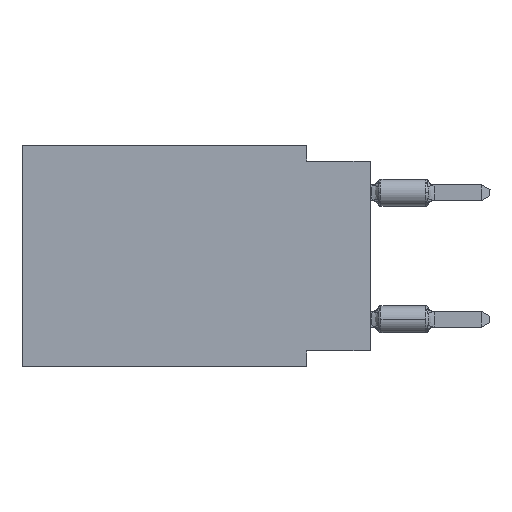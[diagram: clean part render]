
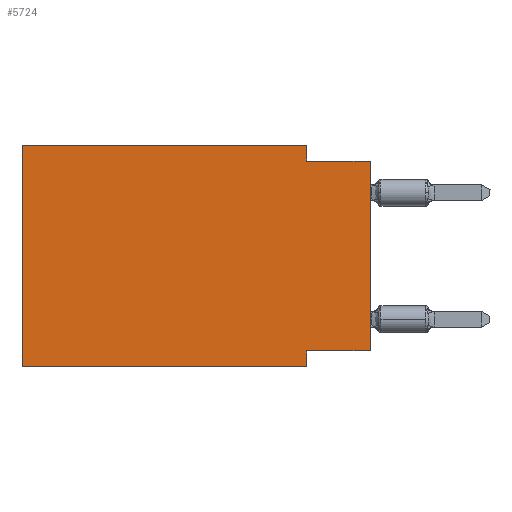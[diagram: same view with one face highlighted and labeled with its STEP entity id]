
A CAD part, left-side view. The second image highlights one B-rep face of the part: STEP entity #5724.
In plain terms, the highlighted planar face has unit normal (-1, 0, 0).
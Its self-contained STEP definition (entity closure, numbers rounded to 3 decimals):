
#1336 = VERTEX_POINT ( 'NONE', #9632 ) ;
#2254 = LINE ( 'NONE', #15727, #28771 ) ;
#2940 = FACE_OUTER_BOUND ( 'NONE', #17958, .T. ) ;
#3119 = ORIENTED_EDGE ( 'NONE', *, *, #3283, .T. ) ;
#3283 = EDGE_CURVE ( 'NONE', #20167, #16165, #27221, .T. ) ;
#3312 = ORIENTED_EDGE ( 'NONE', *, *, #26765, .F. ) ;
#3314 = EDGE_CURVE ( 'NONE', #15516, #1336, #30475, .T. ) ;
#3693 = EDGE_CURVE ( 'NONE', #4203, #21512, #18870, .T. ) ;
#3713 = CARTESIAN_POINT ( 'NONE',  ( 0., 0., -8.255 ) ) ;
#4203 = VERTEX_POINT ( 'NONE', #17099 ) ;
#5093 = DIRECTION ( 'NONE',  ( 0., -1., 0. ) ) ;
#5327 = VECTOR ( 'NONE', #5093, 1000. ) ;
#5641 = EDGE_CURVE ( 'NONE', #21512, #9783, #30757, .T. ) ;
#5724 = ADVANCED_FACE ( 'NONE', ( #2940 ), #10731, .F. ) ;
#7027 = CARTESIAN_POINT ( 'NONE',  ( 0., 2.54, 0. ) ) ;
#7473 = DIRECTION ( 'NONE',  ( 0., -1., 0. ) ) ;
#7504 = VECTOR ( 'NONE', #22390, 1000. ) ;
#7661 = ORIENTED_EDGE ( 'NONE', *, *, #32866, .F. ) ;
#8297 = DIRECTION ( 'NONE',  ( 0., 0., -1. ) ) ;
#9632 = CARTESIAN_POINT ( 'NONE',  ( 0., 2.54, -8.255 ) ) ;
#9783 = VERTEX_POINT ( 'NONE', #26703 ) ;
#10731 = PLANE ( 'NONE',  #22887 ) ;
#11315 = VECTOR ( 'NONE', #22113, 1000. ) ;
#11355 = CARTESIAN_POINT ( 'NONE',  ( 0., 13.97, -8.89 ) ) ;
#11459 = ORIENTED_EDGE ( 'NONE', *, *, #3314, .F. ) ;
#12069 = DIRECTION ( 'NONE',  ( 0., 0., 1. ) ) ;
#12221 = CARTESIAN_POINT ( 'NONE',  ( 0., 0., 0. ) ) ;
#13426 = DIRECTION ( 'NONE',  ( 0., 0., -1. ) ) ;
#13707 = CARTESIAN_POINT ( 'NONE',  ( 0., 13.97, 0. ) ) ;
#14264 = CARTESIAN_POINT ( 'NONE',  ( 0., 0., -8.255 ) ) ;
#14338 = CARTESIAN_POINT ( 'NONE',  ( 0., 13.97, 0. ) ) ;
#15516 = VERTEX_POINT ( 'NONE', #3713 ) ;
#15727 = CARTESIAN_POINT ( 'NONE',  ( 0., 0., -0.635 ) ) ;
#16165 = VERTEX_POINT ( 'NONE', #19003 ) ;
#16587 = LINE ( 'NONE', #14338, #11315 ) ;
#17099 = CARTESIAN_POINT ( 'NONE',  ( 0., 13.97, 0. ) ) ;
#17904 = ORIENTED_EDGE ( 'NONE', *, *, #3693, .F. ) ;
#17958 = EDGE_LOOP ( 'NONE', ( #26863, #3312, #33138, #17904, #29126, #3119, #7661, #11459 ) ) ;
#18870 = LINE ( 'NONE', #13707, #5327 ) ;
#19003 = CARTESIAN_POINT ( 'NONE',  ( 0., 2.54, -8.89 ) ) ;
#19270 = DIRECTION ( 'NONE',  ( 0., 1., 0. ) ) ;
#20006 = EDGE_CURVE ( 'NONE', #15516, #26347, #31041, .T. ) ;
#20167 = VERTEX_POINT ( 'NONE', #26731 ) ;
#20931 = CARTESIAN_POINT ( 'NONE',  ( 0., 0., -0.635 ) ) ;
#21512 = VERTEX_POINT ( 'NONE', #7027 ) ;
#21833 = VECTOR ( 'NONE', #19270, 1000. ) ;
#22113 = DIRECTION ( 'NONE',  ( 0., 0., 1. ) ) ;
#22357 = VECTOR ( 'NONE', #13426, 1000. ) ;
#22390 = DIRECTION ( 'NONE',  ( 0., -1., 0. ) ) ;
#22887 = AXIS2_PLACEMENT_3D ( 'NONE', #29339, #23658, #32106 ) ;
#23429 = VECTOR ( 'NONE', #8297, 1000. ) ;
#23658 = DIRECTION ( 'NONE',  ( 1., 0., 0. ) ) ;
#26347 = VERTEX_POINT ( 'NONE', #20931 ) ;
#26703 = CARTESIAN_POINT ( 'NONE',  ( 0., 2.54, -0.635 ) ) ;
#26731 = CARTESIAN_POINT ( 'NONE',  ( 0., 13.97, -8.89 ) ) ;
#26765 = EDGE_CURVE ( 'NONE', #9783, #26347, #2254, .T. ) ;
#26863 = ORIENTED_EDGE ( 'NONE', *, *, #20006, .T. ) ;
#27126 = VECTOR ( 'NONE', #12069, 1000. ) ;
#27221 = LINE ( 'NONE', #11355, #7504 ) ;
#28771 = VECTOR ( 'NONE', #7473, 1000. ) ;
#29126 = ORIENTED_EDGE ( 'NONE', *, *, #32356, .F. ) ;
#29339 = CARTESIAN_POINT ( 'NONE',  ( 0., 13.97, 0. ) ) ;
#30475 = LINE ( 'NONE', #14264, #21833 ) ;
#30757 = LINE ( 'NONE', #33673, #23429 ) ;
#31041 = LINE ( 'NONE', #12221, #27126 ) ;
#31894 = LINE ( 'NONE', #33992, #22357 ) ;
#32106 = DIRECTION ( 'NONE',  ( 0., 0., -1. ) ) ;
#32356 = EDGE_CURVE ( 'NONE', #20167, #4203, #16587, .T. ) ;
#32866 = EDGE_CURVE ( 'NONE', #1336, #16165, #31894, .T. ) ;
#33138 = ORIENTED_EDGE ( 'NONE', *, *, #5641, .F. ) ;
#33673 = CARTESIAN_POINT ( 'NONE',  ( 0., 2.54, 0. ) ) ;
#33992 = CARTESIAN_POINT ( 'NONE',  ( 0., 2.54, -8.89 ) ) ;
